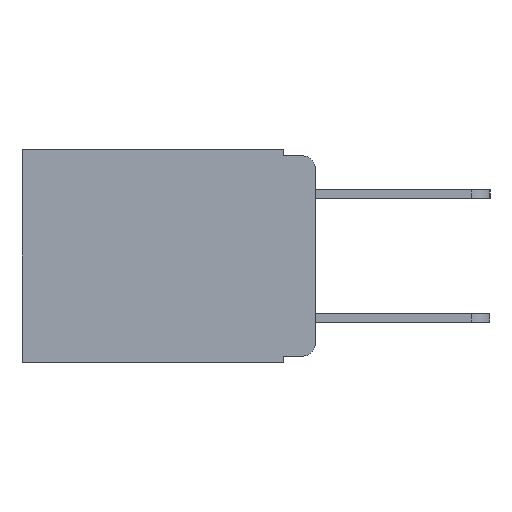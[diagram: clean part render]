
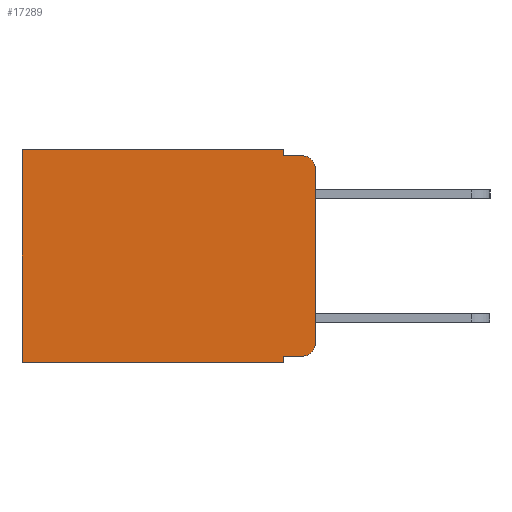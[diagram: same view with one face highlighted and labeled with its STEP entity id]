
A CAD part, left-side view. The second image highlights one B-rep face of the part: STEP entity #17289.
In plain terms, the highlighted planar face has unit normal (-1, 0, 0).
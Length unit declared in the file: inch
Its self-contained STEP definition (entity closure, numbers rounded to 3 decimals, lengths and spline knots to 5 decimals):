
#74 = VECTOR ( 'NONE', #1489, 39.37008 ) ;
#310 = VECTOR ( 'NONE', #16776, 39.37008 ) ;
#1057 = AXIS2_PLACEMENT_3D ( 'NONE', #1090, #13977, #3112 ) ;
#1090 = CARTESIAN_POINT ( 'NONE',  ( 0.298, 0.02, -0.313 ) ) ;
#1278 = ORIENTED_EDGE ( 'NONE', *, *, #11846, .F. ) ;
#1489 = DIRECTION ( 'NONE',  ( 0., 0., -1. ) ) ;
#1582 = ORIENTED_EDGE ( 'NONE', *, *, #20133, .T. ) ;
#2565 = PLANE ( 'NONE',  #16522 ) ;
#3112 = DIRECTION ( 'NONE',  ( 0., 0., -1. ) ) ;
#3456 = ORIENTED_EDGE ( 'NONE', *, *, #5149, .F. ) ;
#3509 = CARTESIAN_POINT ( 'NONE',  ( 0.298, 0., -0.343 ) ) ;
#4046 = VECTOR ( 'NONE', #17511, 39.37008 ) ;
#4244 = VERTEX_POINT ( 'NONE', #8040 ) ;
#4995 = VERTEX_POINT ( 'NONE', #17163 ) ;
#5058 = CARTESIAN_POINT ( 'NONE',  ( 0.298, 0.473, 0. ) ) ;
#5139 = EDGE_CURVE ( 'NONE', #4995, #10155, #8512, .T. ) ;
#5149 = EDGE_CURVE ( 'NONE', #10155, #14290, #17907, .T. ) ;
#5380 = CARTESIAN_POINT ( 'NONE',  ( 0.298, 0.051, 0. ) ) ;
#5667 = VECTOR ( 'NONE', #7744, 39.37008 ) ;
#5813 = EDGE_LOOP ( 'NONE', ( #20968, #19904, #1278, #18826, #19355, #9475, #3456, #13099, #1582, #17213 ) ) ;
#5838 = VERTEX_POINT ( 'NONE', #10963 ) ;
#5973 = EDGE_CURVE ( 'NONE', #9260, #8029, #6803, .T. ) ;
#6450 = DIRECTION ( 'NONE',  ( 0., -1., 0. ) ) ;
#6803 = LINE ( 'NONE', #9548, #5667 ) ;
#6875 = CARTESIAN_POINT ( 'NONE',  ( 0.298, 0.02, -0.03 ) ) ;
#7612 = CARTESIAN_POINT ( 'NONE',  ( 0.298, 0.051, -0.333 ) ) ;
#7744 = DIRECTION ( 'NONE',  ( 0., 1., 0. ) ) ;
#7828 = LINE ( 'NONE', #20549, #21768 ) ;
#8029 = VERTEX_POINT ( 'NONE', #5058 ) ;
#8040 = CARTESIAN_POINT ( 'NONE',  ( 0.298, 0.051, -0.01 ) ) ;
#8173 = DIRECTION ( 'NONE',  ( 0., 0., -1. ) ) ;
#8512 = LINE ( 'NONE', #5380, #9079 ) ;
#8641 = EDGE_CURVE ( 'NONE', #9778, #5838, #9504, .T. ) ;
#8655 = CARTESIAN_POINT ( 'NONE',  ( 0.298, 0.051, -0.343 ) ) ;
#8693 = CIRCLE ( 'NONE', #1057, 0.02 ) ;
#8701 = DIRECTION ( 'NONE',  ( 0., 0., -1. ) ) ;
#8911 = LINE ( 'NONE', #22616, #4046 ) ;
#8971 = CARTESIAN_POINT ( 'NONE',  ( 0.298, 0.02, -0.333 ) ) ;
#9079 = VECTOR ( 'NONE', #17827, 39.37008 ) ;
#9260 = VERTEX_POINT ( 'NONE', #22816 ) ;
#9415 = DIRECTION ( 'NONE',  ( 0., -1., 0. ) ) ;
#9475 = ORIENTED_EDGE ( 'NONE', *, *, #10894, .T. ) ;
#9504 = CIRCLE ( 'NONE', #17412, 0.02 ) ;
#9548 = CARTESIAN_POINT ( 'NONE',  ( 0.298, 0., 0. ) ) ;
#9778 = VERTEX_POINT ( 'NONE', #15641 ) ;
#10155 = VERTEX_POINT ( 'NONE', #8655 ) ;
#10324 = LINE ( 'NONE', #20159, #310 ) ;
#10894 = EDGE_CURVE ( 'NONE', #8029, #14290, #13743, .T. ) ;
#10963 = CARTESIAN_POINT ( 'NONE',  ( 0.298, 0.02, -0.01 ) ) ;
#11707 = CARTESIAN_POINT ( 'NONE',  ( 0.298, 0., -0.313 ) ) ;
#11846 = EDGE_CURVE ( 'NONE', #4244, #5838, #7828, .T. ) ;
#12378 = EDGE_CURVE ( 'NONE', #9260, #4244, #10324, .T. ) ;
#12661 = EDGE_CURVE ( 'NONE', #9778, #16000, #8911, .T. ) ;
#12688 = VECTOR ( 'NONE', #14336, 39.37008 ) ;
#13099 = ORIENTED_EDGE ( 'NONE', *, *, #5139, .F. ) ;
#13743 = LINE ( 'NONE', #21173, #74 ) ;
#13977 = DIRECTION ( 'NONE',  ( -1., 0., 0. ) ) ;
#14290 = VERTEX_POINT ( 'NONE', #19045 ) ;
#14336 = DIRECTION ( 'NONE',  ( 0., 1., 0. ) ) ;
#15641 = CARTESIAN_POINT ( 'NONE',  ( 0.298, 0., -0.03 ) ) ;
#16000 = VERTEX_POINT ( 'NONE', #11707 ) ;
#16007 = LINE ( 'NONE', #7612, #21120 ) ;
#16522 = AXIS2_PLACEMENT_3D ( 'NONE', #20388, #18736, #8173 ) ;
#16776 = DIRECTION ( 'NONE',  ( 0., 0., -1. ) ) ;
#16812 = EDGE_CURVE ( 'NONE', #23110, #16000, #8693, .T. ) ;
#16989 = FACE_OUTER_BOUND ( 'NONE', #5813, .T. ) ;
#17163 = CARTESIAN_POINT ( 'NONE',  ( 0.298, 0.051, -0.333 ) ) ;
#17213 = ORIENTED_EDGE ( 'NONE', *, *, #16812, .T. ) ;
#17289 = ADVANCED_FACE ( 'NONE', ( #16989 ), #2565, .F. ) ;
#17412 = AXIS2_PLACEMENT_3D ( 'NONE', #6875, #19234, #8701 ) ;
#17511 = DIRECTION ( 'NONE',  ( 0., 0., -1. ) ) ;
#17827 = DIRECTION ( 'NONE',  ( 0., 0., -1. ) ) ;
#17907 = LINE ( 'NONE', #3509, #12688 ) ;
#18736 = DIRECTION ( 'NONE',  ( 1., 0., 0. ) ) ;
#18826 = ORIENTED_EDGE ( 'NONE', *, *, #12378, .F. ) ;
#19045 = CARTESIAN_POINT ( 'NONE',  ( 0.298, 0.473, -0.343 ) ) ;
#19234 = DIRECTION ( 'NONE',  ( -1., 0., 0. ) ) ;
#19355 = ORIENTED_EDGE ( 'NONE', *, *, #5973, .T. ) ;
#19904 = ORIENTED_EDGE ( 'NONE', *, *, #8641, .T. ) ;
#20133 = EDGE_CURVE ( 'NONE', #4995, #23110, #16007, .T. ) ;
#20159 = CARTESIAN_POINT ( 'NONE',  ( 0.298, 0.051, 0. ) ) ;
#20388 = CARTESIAN_POINT ( 'NONE',  ( 0.298, 0., 0. ) ) ;
#20549 = CARTESIAN_POINT ( 'NONE',  ( 0.298, 0.051, -0.01 ) ) ;
#20968 = ORIENTED_EDGE ( 'NONE', *, *, #12661, .F. ) ;
#21120 = VECTOR ( 'NONE', #9415, 39.37008 ) ;
#21173 = CARTESIAN_POINT ( 'NONE',  ( 0.298, 0.473, 0. ) ) ;
#21768 = VECTOR ( 'NONE', #6450, 39.37008 ) ;
#22616 = CARTESIAN_POINT ( 'NONE',  ( 0.298, 0., 0. ) ) ;
#22816 = CARTESIAN_POINT ( 'NONE',  ( 0.298, 0.051, 0. ) ) ;
#23110 = VERTEX_POINT ( 'NONE', #8971 ) ;
